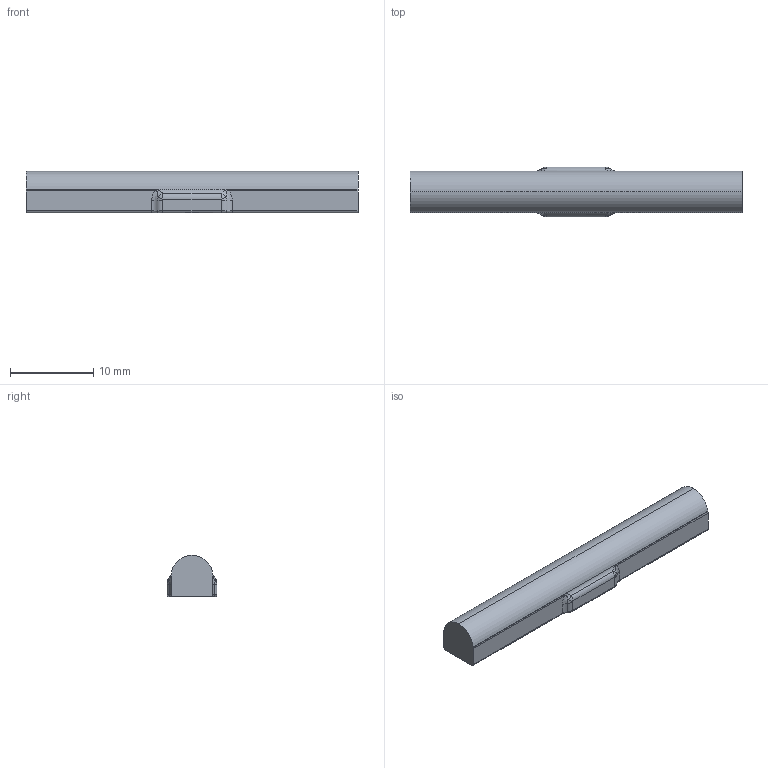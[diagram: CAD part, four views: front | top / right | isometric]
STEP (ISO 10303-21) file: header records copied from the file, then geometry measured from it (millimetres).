
FILE_DESCRIPTION (( 'STEP AP214' ), '1' );
FILE_NAME ('Barrel_Lock_Rod.step', '2013-11-06T14:30:48', ( 'elpi' ), ( '' ), 'SwSTEP 2.0', 'SolidWorks 2013', '' );
FILE_SCHEMA (( 'AUTOMOTIVE_DESIGN' ));
Length unit declared in the file: millimetre
Products named in the file (1): Barrel_Lock_Rod
Bounding box: 40 x 6 x 5 mm (x, y, z)
Volume: 881.7 mm3; surface area: 805.4 mm2
Topology: 1 solids, 1 shells, 68 faces, 163 edges, 94 vertices
Faces by surface type: cylinder 26, torus 12, plane 12, bspline 12, sphere 4, cone 2
Entity records: 2273 total; most frequent: CARTESIAN_POINT 718, DIRECTION 333, ORIENTED_EDGE 318, EDGE_CURVE 159, AXIS2_PLACEMENT_3D 141, VERTEX_POINT 94, CIRCLE 84, EDGE_LOOP 69
